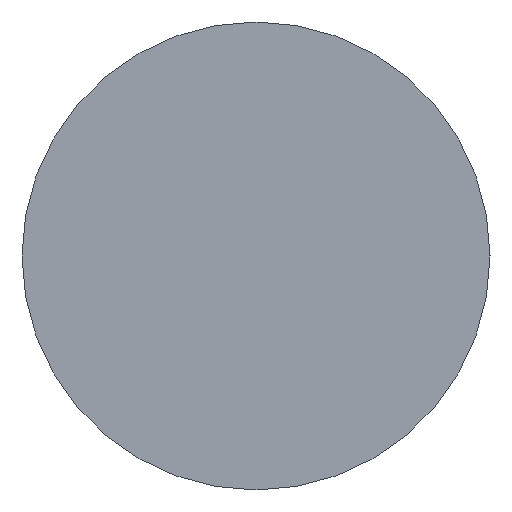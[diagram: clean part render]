
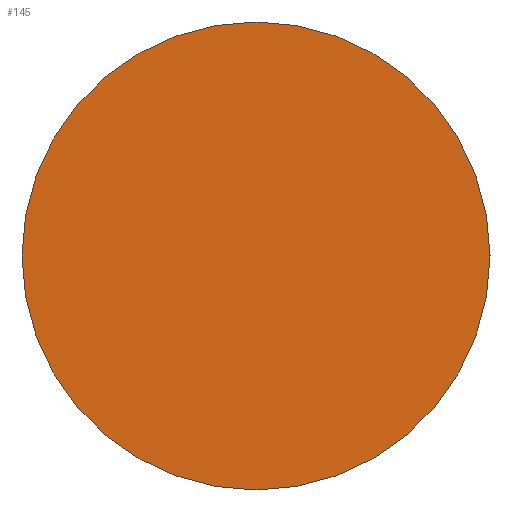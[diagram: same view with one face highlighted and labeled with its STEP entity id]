
A CAD part, left-side view. The second image highlights one B-rep face of the part: STEP entity #145.
In plain terms, the highlighted planar face has unit normal (-1, 0, 0).
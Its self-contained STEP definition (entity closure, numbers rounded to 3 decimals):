
#2 = EDGE_CURVE ( 'NONE', #150, #47, #117, .T. ) ;
#9 = DIRECTION ( 'NONE',  ( 1., 0., 0. ) ) ;
#11 = AXIS2_PLACEMENT_3D ( 'NONE', #209, #177, #194 ) ;
#16 = CIRCLE ( 'NONE', #18, 3.75 ) ;
#18 = AXIS2_PLACEMENT_3D ( 'NONE', #81, #9, #78 ) ;
#19 = AXIS2_PLACEMENT_3D ( 'NONE', #104, #48, #27 ) ;
#27 = DIRECTION ( 'NONE',  ( 0., 0., -1. ) ) ;
#32 = FACE_OUTER_BOUND ( 'NONE', #215, .T. ) ;
#47 = VERTEX_POINT ( 'NONE', #208 ) ;
#48 = DIRECTION ( 'NONE',  ( 1., 0., 0. ) ) ;
#51 = CARTESIAN_POINT ( 'NONE',  ( 4.251, 0., 3.75 ) ) ;
#61 = PLANE ( 'NONE',  #19 ) ;
#78 = DIRECTION ( 'NONE',  ( 0., 0., -1. ) ) ;
#81 = CARTESIAN_POINT ( 'NONE',  ( 4.251, 0., 0. ) ) ;
#104 = CARTESIAN_POINT ( 'NONE',  ( 4.251, 0., 0. ) ) ;
#117 = CIRCLE ( 'NONE', #11, 3.75 ) ;
#128 = ORIENTED_EDGE ( 'NONE', *, *, #205, .F. ) ;
#145 = ADVANCED_FACE ( 'NONE', ( #32 ), #61, .F. ) ;
#150 = VERTEX_POINT ( 'NONE', #51 ) ;
#177 = DIRECTION ( 'NONE',  ( 1., 0., 0. ) ) ;
#194 = DIRECTION ( 'NONE',  ( 0., 0., -1. ) ) ;
#203 = ORIENTED_EDGE ( 'NONE', *, *, #2, .F. ) ;
#205 = EDGE_CURVE ( 'NONE', #47, #150, #16, .T. ) ;
#208 = CARTESIAN_POINT ( 'NONE',  ( 4.251, 0., -3.75 ) ) ;
#209 = CARTESIAN_POINT ( 'NONE',  ( 4.251, 0., 0. ) ) ;
#215 = EDGE_LOOP ( 'NONE', ( #203, #128 ) ) ;
